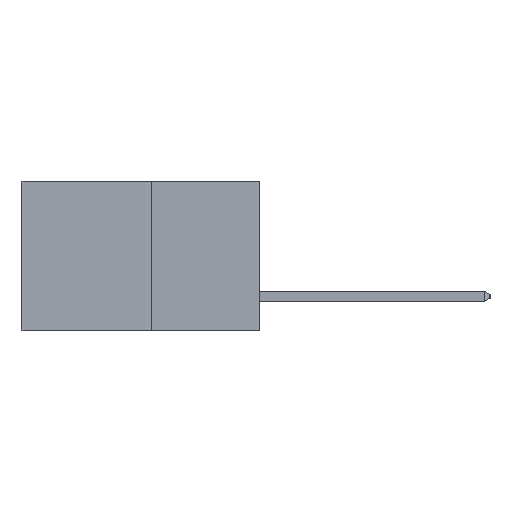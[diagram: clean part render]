
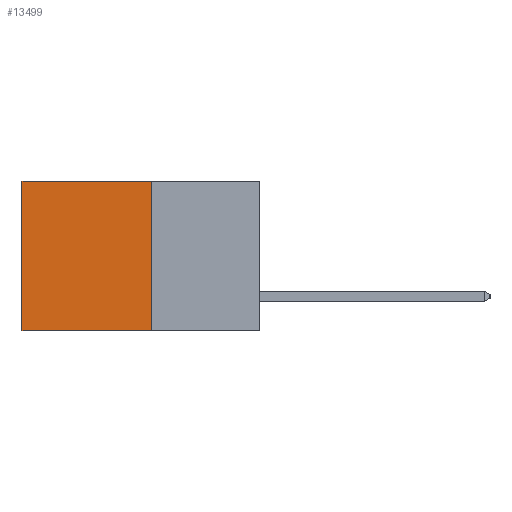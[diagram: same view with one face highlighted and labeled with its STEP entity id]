
A CAD part, left-side view. The second image highlights one B-rep face of the part: STEP entity #13499.
In plain terms, the highlighted planar face has unit normal (-1, 0, 0).
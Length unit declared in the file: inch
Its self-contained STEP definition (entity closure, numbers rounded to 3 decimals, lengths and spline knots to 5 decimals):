
#84 = VERTEX_POINT ( 'NONE', #13753 ) ;
#138 = VECTOR ( 'NONE', #20490, 39.37008 ) ;
#512 = CARTESIAN_POINT ( 'NONE',  ( 0.277, 0.27, 0. ) ) ;
#651 = LINE ( 'NONE', #14569, #138 ) ;
#914 = ORIENTED_EDGE ( 'NONE', *, *, #9438, .T. ) ;
#1314 = DIRECTION ( 'NONE',  ( 1., 0., 0. ) ) ;
#1383 = ORIENTED_EDGE ( 'NONE', *, *, #2422, .T. ) ;
#2176 = ORIENTED_EDGE ( 'NONE', *, *, #4713, .F. ) ;
#2422 = EDGE_CURVE ( 'NONE', #3734, #84, #651, .T. ) ;
#3001 = CARTESIAN_POINT ( 'NONE',  ( 0.277, 0.27, -0.37 ) ) ;
#3409 = VECTOR ( 'NONE', #8007, 39.37008 ) ;
#3734 = VERTEX_POINT ( 'NONE', #20263 ) ;
#4598 = LINE ( 'NONE', #512, #12636 ) ;
#4713 = EDGE_CURVE ( 'NONE', #5520, #84, #12496, .T. ) ;
#5520 = VERTEX_POINT ( 'NONE', #3001 ) ;
#7083 = DIRECTION ( 'NONE',  ( 0., 1., 0. ) ) ;
#8007 = DIRECTION ( 'NONE',  ( 0., 1., 0. ) ) ;
#9438 = EDGE_CURVE ( 'NONE', #17525, #3734, #4598, .T. ) ;
#10338 = CARTESIAN_POINT ( 'NONE',  ( 0.277, 0.27, -0.37 ) ) ;
#11306 = ORIENTED_EDGE ( 'NONE', *, *, #19885, .F. ) ;
#12184 = CARTESIAN_POINT ( 'NONE',  ( 0.277, 0.27, -0.37 ) ) ;
#12496 = LINE ( 'NONE', #10338, #3409 ) ;
#12636 = VECTOR ( 'NONE', #7083, 39.37008 ) ;
#12653 = DIRECTION ( 'NONE',  ( 0., 0., -1. ) ) ;
#13499 = ADVANCED_FACE ( 'NONE', ( #18138 ), #17359, .F. ) ;
#13665 = VECTOR ( 'NONE', #13765, 39.37008 ) ;
#13753 = CARTESIAN_POINT ( 'NONE',  ( 0.277, 0.59, -0.37 ) ) ;
#13765 = DIRECTION ( 'NONE',  ( 0., 0., -1. ) ) ;
#14320 = EDGE_LOOP ( 'NONE', ( #1383, #2176, #11306, #914 ) ) ;
#14569 = CARTESIAN_POINT ( 'NONE',  ( 0.277, 0.59, -0.37 ) ) ;
#17359 = PLANE ( 'NONE',  #20560 ) ;
#17444 = CARTESIAN_POINT ( 'NONE',  ( 0.277, 0.27, 0. ) ) ;
#17525 = VERTEX_POINT ( 'NONE', #17444 ) ;
#17853 = LINE ( 'NONE', #12184, #13665 ) ;
#18138 = FACE_OUTER_BOUND ( 'NONE', #14320, .T. ) ;
#19885 = EDGE_CURVE ( 'NONE', #17525, #5520, #17853, .T. ) ;
#20263 = CARTESIAN_POINT ( 'NONE',  ( 0.277, 0.59, 0. ) ) ;
#20470 = CARTESIAN_POINT ( 'NONE',  ( 0.277, 0.27, -0.37 ) ) ;
#20490 = DIRECTION ( 'NONE',  ( 0., 0., -1. ) ) ;
#20560 = AXIS2_PLACEMENT_3D ( 'NONE', #20470, #1314, #12653 ) ;
